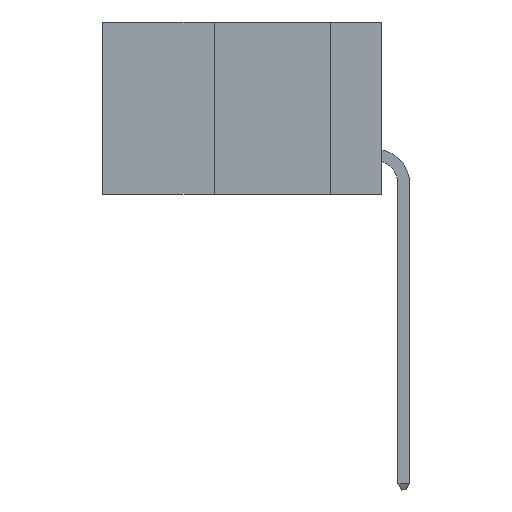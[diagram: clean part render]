
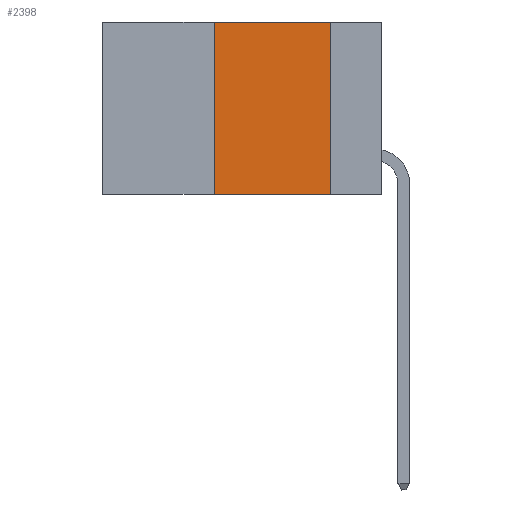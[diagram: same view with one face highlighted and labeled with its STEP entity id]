
A CAD part, left-side view. The second image highlights one B-rep face of the part: STEP entity #2398.
In plain terms, the highlighted planar face has unit normal (-1, 0, 0).
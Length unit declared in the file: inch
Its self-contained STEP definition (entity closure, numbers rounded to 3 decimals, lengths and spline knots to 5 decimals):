
#27 = EDGE_CURVE ( 'NONE', #8693, #9287, #1414, .T. ) ;
#198 = DIRECTION ( 'NONE',  ( 0., -1., 0. ) ) ;
#348 = AXIS2_PLACEMENT_3D ( 'NONE', #3517, #6147, #5305 ) ;
#616 = EDGE_CURVE ( 'NONE', #9966, #9287, #3337, .T. ) ;
#1284 = VECTOR ( 'NONE', #198, 39.37008 ) ;
#1392 = LINE ( 'NONE', #9054, #5040 ) ;
#1414 = LINE ( 'NONE', #5538, #1555 ) ;
#1555 = VECTOR ( 'NONE', #8756, 39.37008 ) ;
#1634 = EDGE_CURVE ( 'NONE', #9966, #3154, #1392, .T. ) ;
#1735 = VECTOR ( 'NONE', #10087, 39.37008 ) ;
#2398 = ADVANCED_FACE ( 'NONE', ( #10283 ), #8655, .F. ) ;
#3030 = CARTESIAN_POINT ( 'NONE',  ( 0., 0.36, -0.37 ) ) ;
#3154 = VERTEX_POINT ( 'NONE', #7339 ) ;
#3163 = ORIENTED_EDGE ( 'NONE', *, *, #1634, .F. ) ;
#3250 = CARTESIAN_POINT ( 'NONE',  ( 0., 0.6, 0. ) ) ;
#3266 = CARTESIAN_POINT ( 'NONE',  ( 0., 0.6, -0.37 ) ) ;
#3337 = LINE ( 'NONE', #3266, #1284 ) ;
#3476 = EDGE_CURVE ( 'NONE', #3154, #8693, #3681, .T. ) ;
#3517 = CARTESIAN_POINT ( 'NONE',  ( 0., 0.6, 0. ) ) ;
#3681 = LINE ( 'NONE', #3250, #1735 ) ;
#3977 = CARTESIAN_POINT ( 'NONE',  ( 0., 0.11, -0.37 ) ) ;
#5040 = VECTOR ( 'NONE', #7428, 39.37008 ) ;
#5305 = DIRECTION ( 'NONE',  ( 0., 0., -1. ) ) ;
#5538 = CARTESIAN_POINT ( 'NONE',  ( 0., 0.11, 0. ) ) ;
#6147 = DIRECTION ( 'NONE',  ( 1., 0., 0. ) ) ;
#6750 = EDGE_LOOP ( 'NONE', ( #8304, #10041, #3163, #9840 ) ) ;
#7339 = CARTESIAN_POINT ( 'NONE',  ( 0., 0.36, 0. ) ) ;
#7428 = DIRECTION ( 'NONE',  ( 0., 0., 1. ) ) ;
#8304 = ORIENTED_EDGE ( 'NONE', *, *, #27, .F. ) ;
#8384 = CARTESIAN_POINT ( 'NONE',  ( 0., 0.11, 0. ) ) ;
#8655 = PLANE ( 'NONE',  #348 ) ;
#8693 = VERTEX_POINT ( 'NONE', #8384 ) ;
#8756 = DIRECTION ( 'NONE',  ( 0., 0., -1. ) ) ;
#9054 = CARTESIAN_POINT ( 'NONE',  ( 0., 0.36, 0. ) ) ;
#9287 = VERTEX_POINT ( 'NONE', #3977 ) ;
#9840 = ORIENTED_EDGE ( 'NONE', *, *, #616, .T. ) ;
#9966 = VERTEX_POINT ( 'NONE', #3030 ) ;
#10041 = ORIENTED_EDGE ( 'NONE', *, *, #3476, .F. ) ;
#10087 = DIRECTION ( 'NONE',  ( 0., -1., 0. ) ) ;
#10283 = FACE_OUTER_BOUND ( 'NONE', #6750, .T. ) ;
